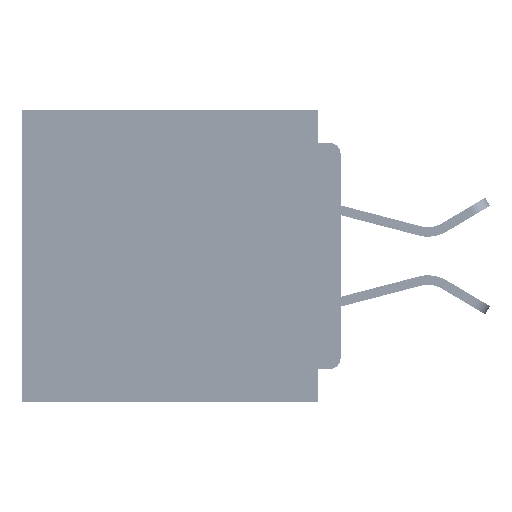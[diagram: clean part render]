
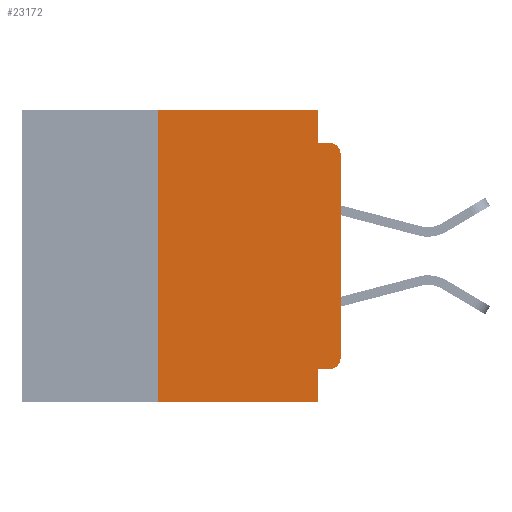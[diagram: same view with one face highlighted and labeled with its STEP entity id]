
A CAD part, left-side view. The second image highlights one B-rep face of the part: STEP entity #23172.
In plain terms, the highlighted planar face has unit normal (-1, 0, 0).
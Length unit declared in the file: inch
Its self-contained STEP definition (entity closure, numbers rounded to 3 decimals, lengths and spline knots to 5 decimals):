
#577 = VECTOR ( 'NONE', #56120, 39.37008 ) ;
#1098 = CARTESIAN_POINT ( 'NONE',  ( 0., 0.25, -0.4 ) ) ;
#1499 = VERTEX_POINT ( 'NONE', #2174 ) ;
#2035 = AXIS2_PLACEMENT_3D ( 'NONE', #46263, #15593, #51397 ) ;
#2174 = CARTESIAN_POINT ( 'NONE',  ( 0., 0., -0.34 ) ) ;
#3067 = VECTOR ( 'NONE', #13825, 39.37008 ) ;
#4481 = CARTESIAN_POINT ( 'NONE',  ( 0., 0.031, -0.355 ) ) ;
#4497 = DIRECTION ( 'NONE',  ( 0., 0., -1. ) ) ;
#4641 = ORIENTED_EDGE ( 'NONE', *, *, #11680, .T. ) ;
#4747 = DIRECTION ( 'NONE',  ( 1., 0., 0. ) ) ;
#5051 = VERTEX_POINT ( 'NONE', #4481 ) ;
#6382 = ORIENTED_EDGE ( 'NONE', *, *, #52829, .F. ) ;
#7436 = ORIENTED_EDGE ( 'NONE', *, *, #21990, .F. ) ;
#8767 = CARTESIAN_POINT ( 'NONE',  ( 0., 0.015, -0.045 ) ) ;
#9034 = CARTESIAN_POINT ( 'NONE',  ( 0., 0.031, -0.4 ) ) ;
#9667 = CARTESIAN_POINT ( 'NONE',  ( 0., 0.031, 0. ) ) ;
#10890 = CIRCLE ( 'NONE', #34466, 0.015 ) ;
#11680 = EDGE_CURVE ( 'NONE', #30681, #25301, #15147, .T. ) ;
#12241 = FACE_OUTER_BOUND ( 'NONE', #30159, .T. ) ;
#12315 = VECTOR ( 'NONE', #25123, 39.37008 ) ;
#13825 = DIRECTION ( 'NONE',  ( 0., -1., 0. ) ) ;
#14199 = DIRECTION ( 'NONE',  ( 0., 0., -1. ) ) ;
#15147 = LINE ( 'NONE', #24151, #3067 ) ;
#15593 = DIRECTION ( 'NONE',  ( -1., 0., 0. ) ) ;
#15935 = CARTESIAN_POINT ( 'NONE',  ( 0., 0.437, 0. ) ) ;
#16621 = VECTOR ( 'NONE', #35324, 39.37008 ) ;
#17801 = ORIENTED_EDGE ( 'NONE', *, *, #20765, .T. ) ;
#18738 = LINE ( 'NONE', #9667, #44401 ) ;
#19155 = CARTESIAN_POINT ( 'NONE',  ( 0., 0., -0.045 ) ) ;
#19690 = VECTOR ( 'NONE', #21098, 39.37008 ) ;
#19821 = LINE ( 'NONE', #30140, #16621 ) ;
#20296 = CARTESIAN_POINT ( 'NONE',  ( 0., 0., -0.355 ) ) ;
#20765 = EDGE_CURVE ( 'NONE', #49528, #39980, #10890, .T. ) ;
#21098 = DIRECTION ( 'NONE',  ( 0., -1., 0. ) ) ;
#21990 = EDGE_CURVE ( 'NONE', #61638, #30188, #18738, .T. ) ;
#21998 = CARTESIAN_POINT ( 'NONE',  ( 0., 0.25, 0. ) ) ;
#22991 = CARTESIAN_POINT ( 'NONE',  ( 0., 0.031, -0.045 ) ) ;
#23172 = ADVANCED_FACE ( 'NONE', ( #12241 ), #35312, .F. ) ;
#24151 = CARTESIAN_POINT ( 'NONE',  ( 0., 0.437, -0.4 ) ) ;
#24330 = DIRECTION ( 'NONE',  ( 0., -1., 0. ) ) ;
#25123 = DIRECTION ( 'NONE',  ( 0., 0., 1. ) ) ;
#25301 = VERTEX_POINT ( 'NONE', #63590 ) ;
#25963 = LINE ( 'NONE', #35249, #12315 ) ;
#26347 = CARTESIAN_POINT ( 'NONE',  ( 0., 0., -0.06 ) ) ;
#26478 = ORIENTED_EDGE ( 'NONE', *, *, #42781, .F. ) ;
#28179 = ORIENTED_EDGE ( 'NONE', *, *, #48135, .F. ) ;
#30140 = CARTESIAN_POINT ( 'NONE',  ( 0., 0., 0. ) ) ;
#30159 = EDGE_LOOP ( 'NONE', ( #35529, #17801, #6382, #7436, #28179, #26478, #4641, #32855, #46945, #47142 ) ) ;
#30188 = VERTEX_POINT ( 'NONE', #22991 ) ;
#30612 = CIRCLE ( 'NONE', #2035, 0.015 ) ;
#30679 = DIRECTION ( 'NONE',  ( -1., 0., 0. ) ) ;
#30681 = VERTEX_POINT ( 'NONE', #1098 ) ;
#32855 = ORIENTED_EDGE ( 'NONE', *, *, #42190, .F. ) ;
#34466 = AXIS2_PLACEMENT_3D ( 'NONE', #61271, #30679, #61307 ) ;
#35115 = CARTESIAN_POINT ( 'NONE',  ( 0., 0.015, -0.355 ) ) ;
#35249 = CARTESIAN_POINT ( 'NONE',  ( 0., 0.25, -0.4 ) ) ;
#35312 = PLANE ( 'NONE',  #48230 ) ;
#35324 = DIRECTION ( 'NONE',  ( 0., 0., 1. ) ) ;
#35504 = EDGE_CURVE ( 'NONE', #39420, #5051, #39986, .T. ) ;
#35529 = ORIENTED_EDGE ( 'NONE', *, *, #47351, .T. ) ;
#36343 = VERTEX_POINT ( 'NONE', #21998 ) ;
#37617 = EDGE_CURVE ( 'NONE', #39420, #1499, #30612, .T. ) ;
#38667 = CARTESIAN_POINT ( 'NONE',  ( 0., 0.031, 0. ) ) ;
#39420 = VERTEX_POINT ( 'NONE', #35115 ) ;
#39980 = VERTEX_POINT ( 'NONE', #8767 ) ;
#39986 = LINE ( 'NONE', #20296, #577 ) ;
#40688 = DIRECTION ( 'NONE',  ( 0., 0., -1. ) ) ;
#42190 = EDGE_CURVE ( 'NONE', #5051, #25301, #62026, .T. ) ;
#42781 = EDGE_CURVE ( 'NONE', #30681, #36343, #25963, .T. ) ;
#44401 = VECTOR ( 'NONE', #4497, 39.37008 ) ;
#46263 = CARTESIAN_POINT ( 'NONE',  ( 0., 0.015, -0.34 ) ) ;
#46922 = LINE ( 'NONE', #15935, #19690 ) ;
#46945 = ORIENTED_EDGE ( 'NONE', *, *, #35504, .F. ) ;
#47142 = ORIENTED_EDGE ( 'NONE', *, *, #37617, .T. ) ;
#47351 = EDGE_CURVE ( 'NONE', #1499, #49528, #19821, .T. ) ;
#48135 = EDGE_CURVE ( 'NONE', #36343, #61638, #46922, .T. ) ;
#48230 = AXIS2_PLACEMENT_3D ( 'NONE', #60942, #4747, #40688 ) ;
#49528 = VERTEX_POINT ( 'NONE', #26347 ) ;
#49746 = VECTOR ( 'NONE', #24330, 39.37008 ) ;
#50874 = VECTOR ( 'NONE', #14199, 39.37008 ) ;
#51397 = DIRECTION ( 'NONE',  ( 0., 0., -1. ) ) ;
#52829 = EDGE_CURVE ( 'NONE', #30188, #39980, #52950, .T. ) ;
#52950 = LINE ( 'NONE', #19155, #49746 ) ;
#56120 = DIRECTION ( 'NONE',  ( 0., 1., 0. ) ) ;
#60942 = CARTESIAN_POINT ( 'NONE',  ( 0., 0.437, 0. ) ) ;
#61271 = CARTESIAN_POINT ( 'NONE',  ( 0., 0.015, -0.06 ) ) ;
#61307 = DIRECTION ( 'NONE',  ( 0., 0., -1. ) ) ;
#61638 = VERTEX_POINT ( 'NONE', #38667 ) ;
#62026 = LINE ( 'NONE', #9034, #50874 ) ;
#63590 = CARTESIAN_POINT ( 'NONE',  ( 0., 0.031, -0.4 ) ) ;
